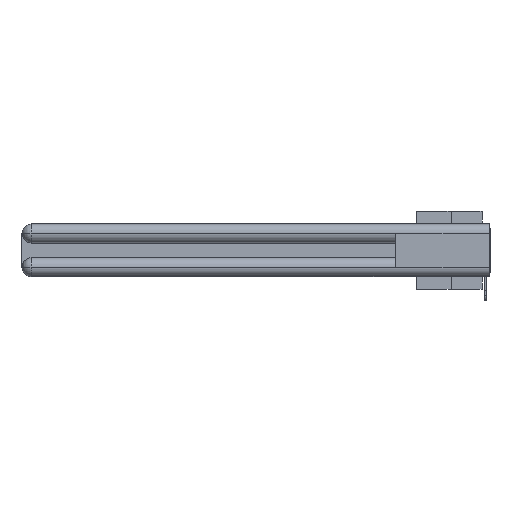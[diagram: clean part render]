
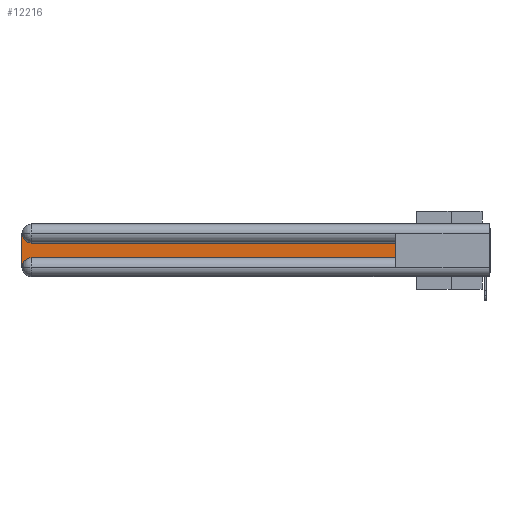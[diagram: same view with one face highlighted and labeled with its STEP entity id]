
A CAD part, left-side view. The second image highlights one B-rep face of the part: STEP entity #12216.
In plain terms, the highlighted planar face has unit normal (-1, 0, 0).
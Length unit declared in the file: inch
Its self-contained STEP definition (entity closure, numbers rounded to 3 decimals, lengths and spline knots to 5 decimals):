
#562 = CARTESIAN_POINT ( 'NONE',  ( 0.075, 0.6, -0.1225 ) ) ;
#643 = EDGE_LOOP ( 'NONE', ( #15751, #17879, #17368, #13334, #5627, #13311 ) ) ;
#683 = DIRECTION ( 'NONE',  ( 0., 0., 1. ) ) ;
#2036 = VERTEX_POINT ( 'NONE', #31993 ) ;
#2135 = CARTESIAN_POINT ( 'NONE',  ( 0.075, 2.94, -0.0625 ) ) ;
#2401 = DIRECTION ( 'NONE',  ( 0., 0., -1. ) ) ;
#4214 = CARTESIAN_POINT ( 'NONE',  ( 0.075, 0.6, -0.2175 ) ) ;
#4322 = DIRECTION ( 'NONE',  ( 1., 0., 0. ) ) ;
#4524 = VERTEX_POINT ( 'NONE', #8594 ) ;
#4770 = LINE ( 'NONE', #21119, #5324 ) ;
#5324 = VECTOR ( 'NONE', #32211, 39.37008 ) ;
#5627 = ORIENTED_EDGE ( 'NONE', *, *, #22209, .T. ) ;
#5737 = EDGE_CURVE ( 'NONE', #34078, #4524, #35257, .T. ) ;
#6374 = LINE ( 'NONE', #562, #24884 ) ;
#7137 = CARTESIAN_POINT ( 'NONE',  ( 0.075, 2.94, -0.2775 ) ) ;
#7344 = PLANE ( 'NONE',  #20275 ) ;
#7537 = FACE_OUTER_BOUND ( 'NONE', #643, .T. ) ;
#8542 = VERTEX_POINT ( 'NONE', #22478 ) ;
#8594 = CARTESIAN_POINT ( 'NONE',  ( 0.075, 3., -0.0625 ) ) ;
#8856 = VERTEX_POINT ( 'NONE', #13548 ) ;
#9687 = AXIS2_PLACEMENT_3D ( 'NONE', #2135, #4322, #18504 ) ;
#10153 = LINE ( 'NONE', #33059, #13266 ) ;
#12216 = ADVANCED_FACE ( 'NONE', ( #7537 ), #7344, .F. ) ;
#12988 = CARTESIAN_POINT ( 'NONE',  ( 0.075, 3., -0.1225 ) ) ;
#13266 = VECTOR ( 'NONE', #24345, 39.37008 ) ;
#13311 = ORIENTED_EDGE ( 'NONE', *, *, #32524, .T. ) ;
#13334 = ORIENTED_EDGE ( 'NONE', *, *, #27310, .T. ) ;
#13548 = CARTESIAN_POINT ( 'NONE',  ( 0.075, 0.6, -0.1225 ) ) ;
#14023 = DIRECTION ( 'NONE',  ( 0., 1., 0. ) ) ;
#15751 = ORIENTED_EDGE ( 'NONE', *, *, #21955, .T. ) ;
#16676 = CARTESIAN_POINT ( 'NONE',  ( 0.075, 0.6, -0.2175 ) ) ;
#17368 = ORIENTED_EDGE ( 'NONE', *, *, #33157, .T. ) ;
#17879 = ORIENTED_EDGE ( 'NONE', *, *, #5737, .T. ) ;
#18440 = DIRECTION ( 'NONE',  ( 1., 0., 0. ) ) ;
#18504 = DIRECTION ( 'NONE',  ( 0., 0., -1. ) ) ;
#20275 = AXIS2_PLACEMENT_3D ( 'NONE', #12988, #18440, #29533 ) ;
#21119 = CARTESIAN_POINT ( 'NONE',  ( 0.075, 3., -0.2175 ) ) ;
#21678 = DIRECTION ( 'NONE',  ( 1., 0., 0. ) ) ;
#21955 = EDGE_CURVE ( 'NONE', #8856, #34078, #6374, .T. ) ;
#22209 = EDGE_CURVE ( 'NONE', #8542, #35618, #10153, .T. ) ;
#22478 = CARTESIAN_POINT ( 'NONE',  ( 0.075, 2.94, -0.2175 ) ) ;
#24345 = DIRECTION ( 'NONE',  ( 0., -1., 0. ) ) ;
#24884 = VECTOR ( 'NONE', #14023, 39.37008 ) ;
#27310 = EDGE_CURVE ( 'NONE', #2036, #8542, #33505, .T. ) ;
#29533 = DIRECTION ( 'NONE',  ( 0., 0., -1. ) ) ;
#30575 = CARTESIAN_POINT ( 'NONE',  ( 0.075, 2.94, -0.1225 ) ) ;
#30687 = LINE ( 'NONE', #16676, #32010 ) ;
#31993 = CARTESIAN_POINT ( 'NONE',  ( 0.075, 3., -0.2775 ) ) ;
#32010 = VECTOR ( 'NONE', #683, 39.37008 ) ;
#32211 = DIRECTION ( 'NONE',  ( 0., 0., -1. ) ) ;
#32524 = EDGE_CURVE ( 'NONE', #35618, #8856, #30687, .T. ) ;
#32901 = AXIS2_PLACEMENT_3D ( 'NONE', #7137, #21678, #2401 ) ;
#33059 = CARTESIAN_POINT ( 'NONE',  ( 0.075, 0.6, -0.2175 ) ) ;
#33157 = EDGE_CURVE ( 'NONE', #4524, #2036, #4770, .T. ) ;
#33505 = CIRCLE ( 'NONE', #32901, 0.06 ) ;
#34078 = VERTEX_POINT ( 'NONE', #30575 ) ;
#35257 = CIRCLE ( 'NONE', #9687, 0.06 ) ;
#35618 = VERTEX_POINT ( 'NONE', #4214 ) ;
